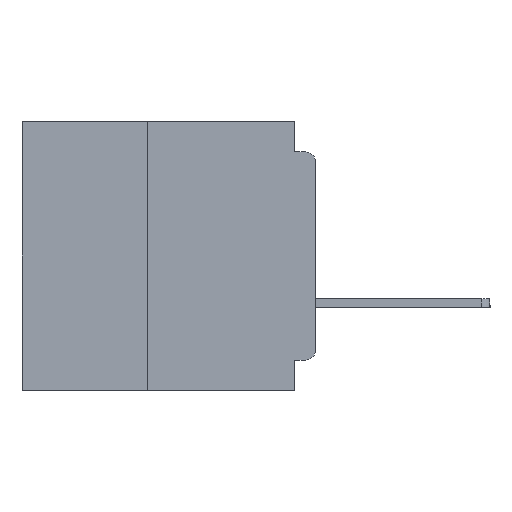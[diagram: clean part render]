
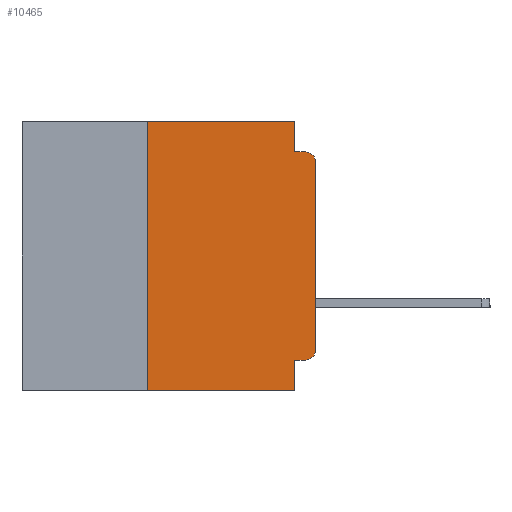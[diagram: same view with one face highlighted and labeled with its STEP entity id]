
A CAD part, left-side view. The second image highlights one B-rep face of the part: STEP entity #10465.
In plain terms, the highlighted planar face has unit normal (-1, 0, 0).
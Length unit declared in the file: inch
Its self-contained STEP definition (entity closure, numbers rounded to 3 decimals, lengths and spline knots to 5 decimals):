
#795 = DIRECTION ( 'NONE',  ( 0., 0., -1. ) ) ;
#798 = EDGE_CURVE ( 'NONE', #28191, #37499, #5760, .T. ) ;
#1067 = EDGE_CURVE ( 'NONE', #9205, #54259, #43124, .T. ) ;
#1204 = EDGE_CURVE ( 'NONE', #24984, #54259, #46968, .T. ) ;
#2861 = DIRECTION ( 'NONE',  ( 0., -1., 0. ) ) ;
#3217 = VECTOR ( 'NONE', #5752, 39.37008 ) ;
#3575 = AXIS2_PLACEMENT_3D ( 'NONE', #21896, #55828, #26768 ) ;
#4567 = VERTEX_POINT ( 'NONE', #40971 ) ;
#5752 = DIRECTION ( 'NONE',  ( 0., 0., -1. ) ) ;
#5760 = LINE ( 'NONE', #21282, #56011 ) ;
#5808 = CARTESIAN_POINT ( 'NONE',  ( 0., 0., -0.045 ) ) ;
#8613 = DIRECTION ( 'NONE',  ( 0., -1., 0. ) ) ;
#9205 = VERTEX_POINT ( 'NONE', #60801 ) ;
#9335 = VERTEX_POINT ( 'NONE', #18168 ) ;
#9642 = VECTOR ( 'NONE', #2861, 39.37008 ) ;
#10465 = ADVANCED_FACE ( 'NONE', ( #22442 ), #54027, .F. ) ;
#11244 = DIRECTION ( 'NONE',  ( 0., 0., -1. ) ) ;
#11591 = CARTESIAN_POINT ( 'NONE',  ( 0., 0., -0.355 ) ) ;
#13030 = ORIENTED_EDGE ( 'NONE', *, *, #1067, .T. ) ;
#15692 = ORIENTED_EDGE ( 'NONE', *, *, #51097, .F. ) ;
#16391 = EDGE_CURVE ( 'NONE', #9335, #37499, #42044, .T. ) ;
#16462 = LINE ( 'NONE', #56118, #37698 ) ;
#17549 = DIRECTION ( 'NONE',  ( 0., 0., 1. ) ) ;
#18168 = CARTESIAN_POINT ( 'NONE',  ( 0., 0.031, -0.355 ) ) ;
#18184 = ORIENTED_EDGE ( 'NONE', *, *, #23306, .F. ) ;
#21282 = CARTESIAN_POINT ( 'NONE',  ( 0., 0.437, -0.4 ) ) ;
#21896 = CARTESIAN_POINT ( 'NONE',  ( 0., 0.015, -0.34 ) ) ;
#22442 = FACE_OUTER_BOUND ( 'NONE', #34110, .T. ) ;
#23175 = DIRECTION ( 'NONE',  ( -1., 0., 0. ) ) ;
#23306 = EDGE_CURVE ( 'NONE', #53311, #9335, #51029, .T. ) ;
#23307 = CARTESIAN_POINT ( 'NONE',  ( 0., 0.015, -0.06 ) ) ;
#24095 = VECTOR ( 'NONE', #29528, 39.37008 ) ;
#24460 = LINE ( 'NONE', #41935, #35809 ) ;
#24984 = VERTEX_POINT ( 'NONE', #58821 ) ;
#25220 = VECTOR ( 'NONE', #50693, 39.37008 ) ;
#26768 = DIRECTION ( 'NONE',  ( 0., 0., -1. ) ) ;
#26916 = ORIENTED_EDGE ( 'NONE', *, *, #798, .T. ) ;
#28191 = VERTEX_POINT ( 'NONE', #61037 ) ;
#28364 = VERTEX_POINT ( 'NONE', #49137 ) ;
#28581 = CARTESIAN_POINT ( 'NONE',  ( 0., 0.015, -0.355 ) ) ;
#29528 = DIRECTION ( 'NONE',  ( 0., 0., 1. ) ) ;
#30032 = DIRECTION ( 'NONE',  ( 1., 0., 0. ) ) ;
#34110 = EDGE_LOOP ( 'NONE', ( #58330, #13030, #61335, #15692, #57360, #58195, #26916, #51694, #18184, #45026 ) ) ;
#35809 = VECTOR ( 'NONE', #46872, 39.37008 ) ;
#37147 = CARTESIAN_POINT ( 'NONE',  ( 0., 0.015, -0.045 ) ) ;
#37499 = VERTEX_POINT ( 'NONE', #52929 ) ;
#37698 = VECTOR ( 'NONE', #41445, 39.37008 ) ;
#40971 = CARTESIAN_POINT ( 'NONE',  ( 0., 0.031, 0. ) ) ;
#41445 = DIRECTION ( 'NONE',  ( 0., 0., -1. ) ) ;
#41717 = CARTESIAN_POINT ( 'NONE',  ( 0., 0.25, -0.4 ) ) ;
#41935 = CARTESIAN_POINT ( 'NONE',  ( 0., 0.437, 0. ) ) ;
#42044 = LINE ( 'NONE', #44698, #3217 ) ;
#43124 = CIRCLE ( 'NONE', #54236, 0.015 ) ;
#43931 = CARTESIAN_POINT ( 'NONE',  ( 0., 0., 0. ) ) ;
#44698 = CARTESIAN_POINT ( 'NONE',  ( 0., 0.031, -0.4 ) ) ;
#45026 = ORIENTED_EDGE ( 'NONE', *, *, #48757, .T. ) ;
#46872 = DIRECTION ( 'NONE',  ( 0., -1., 0. ) ) ;
#46968 = LINE ( 'NONE', #5808, #9642 ) ;
#48757 = EDGE_CURVE ( 'NONE', #53311, #61970, #63070, .T. ) ;
#49137 = CARTESIAN_POINT ( 'NONE',  ( 0., 0.25, 0. ) ) ;
#50693 = DIRECTION ( 'NONE',  ( 0., 1., 0. ) ) ;
#51029 = LINE ( 'NONE', #11591, #25220 ) ;
#51097 = EDGE_CURVE ( 'NONE', #4567, #24984, #16462, .T. ) ;
#51694 = ORIENTED_EDGE ( 'NONE', *, *, #16391, .F. ) ;
#52929 = CARTESIAN_POINT ( 'NONE',  ( 0., 0.031, -0.4 ) ) ;
#53311 = VERTEX_POINT ( 'NONE', #28581 ) ;
#54027 = PLANE ( 'NONE',  #55133 ) ;
#54043 = EDGE_CURVE ( 'NONE', #61970, #9205, #61258, .T. ) ;
#54236 = AXIS2_PLACEMENT_3D ( 'NONE', #23307, #23175, #11244 ) ;
#54259 = VERTEX_POINT ( 'NONE', #37147 ) ;
#54909 = EDGE_CURVE ( 'NONE', #28191, #28364, #58107, .T. ) ;
#55133 = AXIS2_PLACEMENT_3D ( 'NONE', #59107, #30032, #795 ) ;
#55828 = DIRECTION ( 'NONE',  ( -1., 0., 0. ) ) ;
#56011 = VECTOR ( 'NONE', #8613, 39.37008 ) ;
#56118 = CARTESIAN_POINT ( 'NONE',  ( 0., 0.031, 0. ) ) ;
#56594 = VECTOR ( 'NONE', #17549, 39.37008 ) ;
#56771 = EDGE_CURVE ( 'NONE', #28364, #4567, #24460, .T. ) ;
#57360 = ORIENTED_EDGE ( 'NONE', *, *, #56771, .F. ) ;
#58107 = LINE ( 'NONE', #41717, #56594 ) ;
#58195 = ORIENTED_EDGE ( 'NONE', *, *, #54909, .F. ) ;
#58330 = ORIENTED_EDGE ( 'NONE', *, *, #54043, .T. ) ;
#58821 = CARTESIAN_POINT ( 'NONE',  ( 0., 0.031, -0.045 ) ) ;
#59107 = CARTESIAN_POINT ( 'NONE',  ( 0., 0.437, 0. ) ) ;
#60166 = CARTESIAN_POINT ( 'NONE',  ( 0., 0., -0.34 ) ) ;
#60801 = CARTESIAN_POINT ( 'NONE',  ( 0., 0., -0.06 ) ) ;
#61037 = CARTESIAN_POINT ( 'NONE',  ( 0., 0.25, -0.4 ) ) ;
#61258 = LINE ( 'NONE', #43931, #24095 ) ;
#61335 = ORIENTED_EDGE ( 'NONE', *, *, #1204, .F. ) ;
#61970 = VERTEX_POINT ( 'NONE', #60166 ) ;
#63070 = CIRCLE ( 'NONE', #3575, 0.015 ) ;
